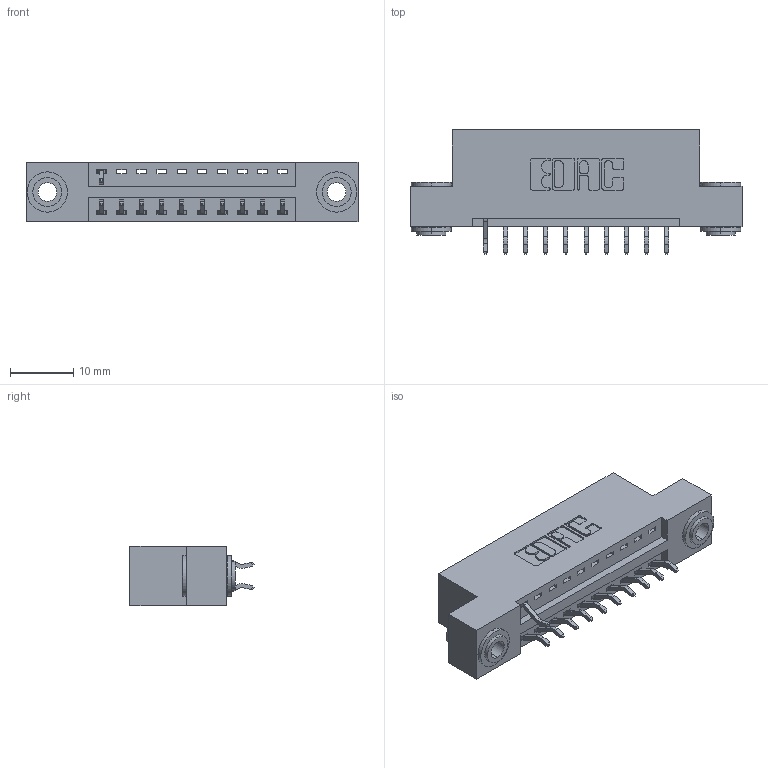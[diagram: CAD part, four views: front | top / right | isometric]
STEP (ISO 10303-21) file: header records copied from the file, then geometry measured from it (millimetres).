
FILE_DESCRIPTION (( 'STEP AP203' ), '1' );
FILE_NAME ('346-020-556-203.STEP', '2018-08-20T22:01:10', ( '' ), ( '' ), 'SwSTEP 2.0', 'SolidWorks 2016', '' );
FILE_SCHEMA (( 'CONFIG_CONTROL_DESIGN' ));
Length unit declared in the file: inch
Products named in the file (4): 346 Part_Flush Mounting Lugs - 0.156 Dia-TH; 345-292-001_556 Tail; 345-250-002_345-250-002-102; 346-020-556-203
Assembly tree (14 placements, depth 2):
  346-020-556-203
    346 Part_Flush Mounting Lugs - 0.156 Dia-TH
    345-292-001_556 Tail  x11
    345-250-002_345-250-002-102  x2
Bounding box: 52.32 x 19.57 x 9.4 mm (x, y, z)
Volume: 4791.7 mm3; surface area: 5820.4 mm2
Topology: 14 solids, 14 shells, 852 faces, 2497 edges, 1646 vertices
Faces by surface type: plane 560, cylinder 284, cone 8
Entity records: 11416 total; most frequent: CARTESIAN_POINT 1954, ORIENTED_EDGE 1878, DIRECTION 1783, EDGE_CURVE 939, LINE 735, VECTOR 735, VERTEX_POINT 622, AXIS2_PLACEMENT_3D 524
